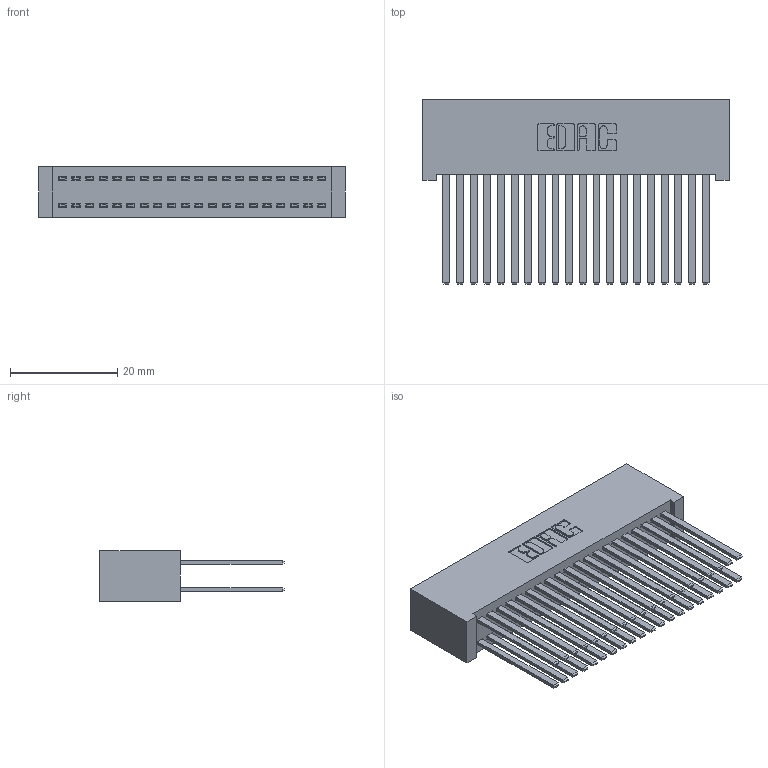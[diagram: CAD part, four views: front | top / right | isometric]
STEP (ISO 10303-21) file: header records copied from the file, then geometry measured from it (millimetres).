
FILE_DESCRIPTION (( 'STEP AP203' ), '1' );
FILE_NAME ('342-040-544-201.STEP', '2019-10-02T16:56:20', ( '' ), ( '' ), 'SwSTEP 2.0', 'SolidWorks 2016', '' );
FILE_SCHEMA (( 'CONFIG_CONTROL_DESIGN' ));
Length unit declared in the file: inch
Products named in the file (3): 345-292-001_345-293-144; 342-040-544-201; 342 Part_Lugless
Assembly tree (41 placements, depth 2):
  342-040-544-201
    342 Part_Lugless
    345-292-001_345-293-144  x40
Bounding box: 57.05 x 34.3 x 9.4 mm (x, y, z)
Volume: 6021.9 mm3; surface area: 11259.1 mm2
Topology: 41 solids, 41 shells, 1942 faces, 5755 edges, 3782 vertices
Faces by surface type: plane 1342, cylinder 600
Entity records: 15119 total; most frequent: CARTESIAN_POINT 2526, ORIENTED_EDGE 2462, DIRECTION 2187, EDGE_CURVE 1231, VECTOR 1115, LINE 1115, VERTEX_POINT 818, AXIS2_PLACEMENT_3D 536
